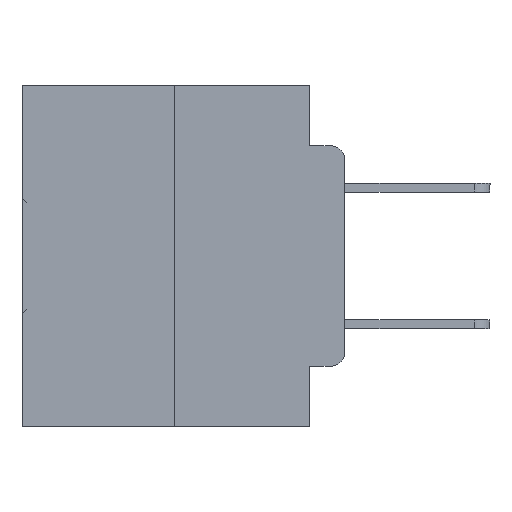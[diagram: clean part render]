
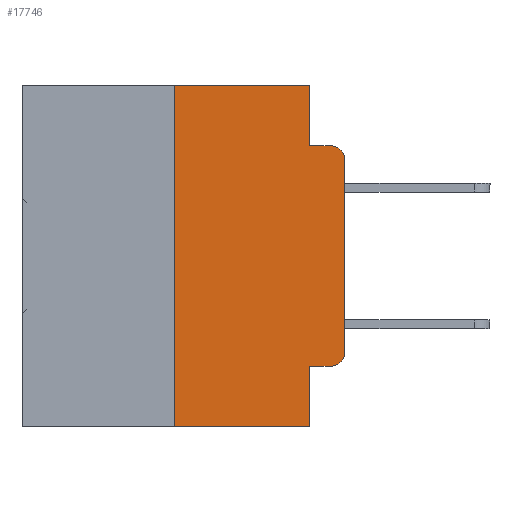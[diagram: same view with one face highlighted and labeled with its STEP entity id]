
A CAD part, left-side view. The second image highlights one B-rep face of the part: STEP entity #17746.
In plain terms, the highlighted planar face has unit normal (-1, 0, 0).
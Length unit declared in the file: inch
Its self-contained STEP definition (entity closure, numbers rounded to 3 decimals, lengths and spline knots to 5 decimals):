
#1788 = VECTOR ( 'NONE', #30311, 39.37008 ) ;
#1964 = LINE ( 'NONE', #22742, #14758 ) ;
#2501 = CARTESIAN_POINT ( 'NONE',  ( 0., 0.25, 0. ) ) ;
#2937 = CARTESIAN_POINT ( 'NONE',  ( 0., 0.051, -0.0885 ) ) ;
#2996 = DIRECTION ( 'NONE',  ( 0., -1., 0. ) ) ;
#3013 = ORIENTED_EDGE ( 'NONE', *, *, #8637, .T. ) ;
#3646 = CARTESIAN_POINT ( 'NONE',  ( 0., 0., 0. ) ) ;
#3923 = CARTESIAN_POINT ( 'NONE',  ( 0., 0., -0.1085 ) ) ;
#4004 = VERTEX_POINT ( 'NONE', #2937 ) ;
#4597 = VECTOR ( 'NONE', #15345, 39.37008 ) ;
#4638 = EDGE_CURVE ( 'NONE', #6482, #6960, #10683, .T. ) ;
#5095 = VECTOR ( 'NONE', #13468, 39.37008 ) ;
#5227 = EDGE_CURVE ( 'NONE', #31002, #10814, #25974, .T. ) ;
#5488 = EDGE_LOOP ( 'NONE', ( #3013, #5838, #5925, #7238, #10815, #10878, #11025, #11493, #11744, #12719 ) ) ;
#5838 = ORIENTED_EDGE ( 'NONE', *, *, #19839, .T. ) ;
#5925 = ORIENTED_EDGE ( 'NONE', *, *, #30520, .F. ) ;
#6244 = VERTEX_POINT ( 'NONE', #24195 ) ;
#6482 = VERTEX_POINT ( 'NONE', #25088 ) ;
#6960 = VERTEX_POINT ( 'NONE', #14591 ) ;
#7146 = EDGE_CURVE ( 'NONE', #12415, #31002, #12142, .T. ) ;
#7238 = ORIENTED_EDGE ( 'NONE', *, *, #13000, .F. ) ;
#7569 = EDGE_CURVE ( 'NONE', #12415, #6244, #18814, .T. ) ;
#8637 = EDGE_CURVE ( 'NONE', #10814, #20549, #21077, .T. ) ;
#8662 = DIRECTION ( 'NONE',  ( 0., 0., 1. ) ) ;
#9221 = PLANE ( 'NONE',  #26549 ) ;
#10063 = VERTEX_POINT ( 'NONE', #12998 ) ;
#10683 = LINE ( 'NONE', #25638, #29198 ) ;
#10814 = VERTEX_POINT ( 'NONE', #18334 ) ;
#10815 = ORIENTED_EDGE ( 'NONE', *, *, #4638, .F. ) ;
#10878 = ORIENTED_EDGE ( 'NONE', *, *, #16742, .F. ) ;
#10979 = VERTEX_POINT ( 'NONE', #16383 ) ;
#11012 = CARTESIAN_POINT ( 'NONE',  ( 0., 0.051, 0. ) ) ;
#11025 = ORIENTED_EDGE ( 'NONE', *, *, #11363, .T. ) ;
#11363 = EDGE_CURVE ( 'NONE', #10979, #6244, #1964, .T. ) ;
#11493 = ORIENTED_EDGE ( 'NONE', *, *, #7569, .F. ) ;
#11744 = ORIENTED_EDGE ( 'NONE', *, *, #7146, .T. ) ;
#11774 = DIRECTION ( 'NONE',  ( 1., 0., 0. ) ) ;
#12110 = VECTOR ( 'NONE', #17041, 39.37008 ) ;
#12142 = LINE ( 'NONE', #12758, #4597 ) ;
#12415 = VERTEX_POINT ( 'NONE', #23436 ) ;
#12719 = ORIENTED_EDGE ( 'NONE', *, *, #5227, .T. ) ;
#12758 = CARTESIAN_POINT ( 'NONE',  ( 0., 0.051, -0.4115 ) ) ;
#12991 = CARTESIAN_POINT ( 'NONE',  ( 0., 0.02, -0.3915 ) ) ;
#12998 = CARTESIAN_POINT ( 'NONE',  ( 0., 0.02, -0.0885 ) ) ;
#13000 = EDGE_CURVE ( 'NONE', #6960, #4004, #19283, .T. ) ;
#13468 = DIRECTION ( 'NONE',  ( 0., -1., 0. ) ) ;
#13824 = AXIS2_PLACEMENT_3D ( 'NONE', #13903, #31409, #16436 ) ;
#13903 = CARTESIAN_POINT ( 'NONE',  ( 0., 0.02, -0.1085 ) ) ;
#14591 = CARTESIAN_POINT ( 'NONE',  ( 0., 0.051, 0. ) ) ;
#14758 = VECTOR ( 'NONE', #20238, 39.37008 ) ;
#15345 = DIRECTION ( 'NONE',  ( 0., -1., 0. ) ) ;
#15564 = DIRECTION ( 'NONE',  ( 0., 0., -1. ) ) ;
#16061 = VECTOR ( 'NONE', #8662, 39.37008 ) ;
#16383 = CARTESIAN_POINT ( 'NONE',  ( 0., 0.25, -0.5 ) ) ;
#16436 = DIRECTION ( 'NONE',  ( 0., 0., -1. ) ) ;
#16742 = EDGE_CURVE ( 'NONE', #10979, #6482, #29474, .T. ) ;
#17041 = DIRECTION ( 'NONE',  ( 0., 0., -1. ) ) ;
#17746 = ADVANCED_FACE ( 'NONE', ( #29796 ), #9221, .F. ) ;
#18121 = AXIS2_PLACEMENT_3D ( 'NONE', #12991, #30538, #15564 ) ;
#18334 = CARTESIAN_POINT ( 'NONE',  ( 0., 0., -0.3915 ) ) ;
#18814 = LINE ( 'NONE', #26982, #12110 ) ;
#19283 = LINE ( 'NONE', #11012, #30288 ) ;
#19839 = EDGE_CURVE ( 'NONE', #20549, #10063, #31196, .T. ) ;
#20238 = DIRECTION ( 'NONE',  ( 0., -1., 0. ) ) ;
#20549 = VERTEX_POINT ( 'NONE', #3923 ) ;
#21077 = LINE ( 'NONE', #3646, #16061 ) ;
#21761 = CARTESIAN_POINT ( 'NONE',  ( 0., 0.473, 0. ) ) ;
#22742 = CARTESIAN_POINT ( 'NONE',  ( 0., 0.473, -0.5 ) ) ;
#23436 = CARTESIAN_POINT ( 'NONE',  ( 0., 0.051, -0.4115 ) ) ;
#23634 = DIRECTION ( 'NONE',  ( 0., 0., -1. ) ) ;
#24195 = CARTESIAN_POINT ( 'NONE',  ( 0., 0.051, -0.5 ) ) ;
#25088 = CARTESIAN_POINT ( 'NONE',  ( 0., 0.25, 0. ) ) ;
#25231 = LINE ( 'NONE', #28508, #5095 ) ;
#25638 = CARTESIAN_POINT ( 'NONE',  ( 0., 0.473, 0. ) ) ;
#25974 = CIRCLE ( 'NONE', #18121, 0.02 ) ;
#26549 = AXIS2_PLACEMENT_3D ( 'NONE', #21761, #11774, #29397 ) ;
#26982 = CARTESIAN_POINT ( 'NONE',  ( 0., 0.051, 0. ) ) ;
#28508 = CARTESIAN_POINT ( 'NONE',  ( 0., 0.051, -0.0885 ) ) ;
#29198 = VECTOR ( 'NONE', #2996, 39.37008 ) ;
#29397 = DIRECTION ( 'NONE',  ( 0., 0., -1. ) ) ;
#29474 = LINE ( 'NONE', #2501, #1788 ) ;
#29796 = FACE_OUTER_BOUND ( 'NONE', #5488, .T. ) ;
#30206 = CARTESIAN_POINT ( 'NONE',  ( 0., 0.02, -0.4115 ) ) ;
#30288 = VECTOR ( 'NONE', #23634, 39.37008 ) ;
#30311 = DIRECTION ( 'NONE',  ( 0., 0., 1. ) ) ;
#30520 = EDGE_CURVE ( 'NONE', #4004, #10063, #25231, .T. ) ;
#30538 = DIRECTION ( 'NONE',  ( -1., 0., 0. ) ) ;
#31002 = VERTEX_POINT ( 'NONE', #30206 ) ;
#31196 = CIRCLE ( 'NONE', #13824, 0.02 ) ;
#31409 = DIRECTION ( 'NONE',  ( -1., 0., 0. ) ) ;
